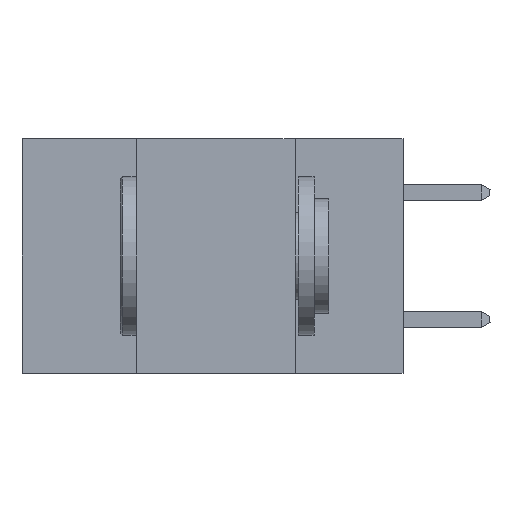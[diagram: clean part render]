
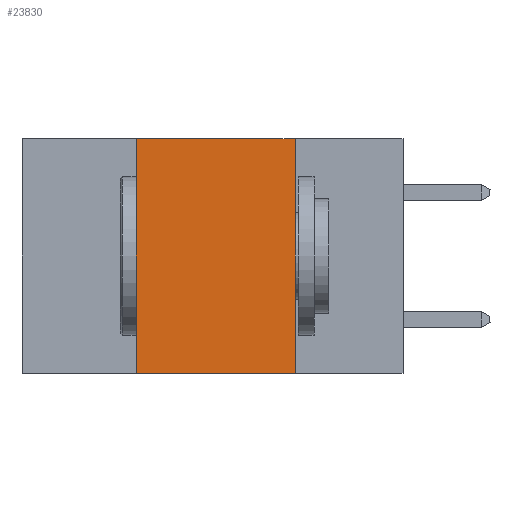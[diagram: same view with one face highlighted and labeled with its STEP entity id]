
A CAD part, left-side view. The second image highlights one B-rep face of the part: STEP entity #23830.
In plain terms, the highlighted planar face has unit normal (-1, 0, 0).
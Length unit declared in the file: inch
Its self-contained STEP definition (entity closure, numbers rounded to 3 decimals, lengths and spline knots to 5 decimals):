
#4 = ORIENTED_EDGE ( 'NONE', *, *, #18553, .F. ) ;
#138 = VECTOR ( 'NONE', #7276, 39.37008 ) ;
#369 = CARTESIAN_POINT ( 'NONE',  ( 0., 0.6, 0. ) ) ;
#420 = CARTESIAN_POINT ( 'NONE',  ( 0., 0.17, -0.37 ) ) ;
#620 = ORIENTED_EDGE ( 'NONE', *, *, #16560, .F. ) ;
#882 = AXIS2_PLACEMENT_3D ( 'NONE', #369, #13523, #2316 ) ;
#1953 = DIRECTION ( 'NONE',  ( 0., 0., -1. ) ) ;
#2316 = DIRECTION ( 'NONE',  ( 0., 0., -1. ) ) ;
#2868 = LINE ( 'NONE', #19048, #3470 ) ;
#3470 = VECTOR ( 'NONE', #17122, 39.37008 ) ;
#3938 = CARTESIAN_POINT ( 'NONE',  ( 0., 0.42, 0. ) ) ;
#5701 = ORIENTED_EDGE ( 'NONE', *, *, #21116, .F. ) ;
#7008 = CARTESIAN_POINT ( 'NONE',  ( 0., 0.42, -0.37 ) ) ;
#7276 = DIRECTION ( 'NONE',  ( 0., 0., 1. ) ) ;
#9091 = VERTEX_POINT ( 'NONE', #7008 ) ;
#9816 = PLANE ( 'NONE',  #882 ) ;
#12121 = VERTEX_POINT ( 'NONE', #19493 ) ;
#13065 = EDGE_LOOP ( 'NONE', ( #4, #620, #5701, #20998 ) ) ;
#13105 = CARTESIAN_POINT ( 'NONE',  ( 0., 0.17, 0. ) ) ;
#13523 = DIRECTION ( 'NONE',  ( 1., 0., 0. ) ) ;
#13578 = FACE_OUTER_BOUND ( 'NONE', #13065, .T. ) ;
#13583 = LINE ( 'NONE', #15158, #22710 ) ;
#13799 = VERTEX_POINT ( 'NONE', #3938 ) ;
#14712 = CARTESIAN_POINT ( 'NONE',  ( 0., 0.42, 0. ) ) ;
#15158 = CARTESIAN_POINT ( 'NONE',  ( 0., 0.6, 0. ) ) ;
#15700 = LINE ( 'NONE', #14712, #138 ) ;
#16560 = EDGE_CURVE ( 'NONE', #13799, #12121, #13583, .T. ) ;
#16988 = DIRECTION ( 'NONE',  ( 0., -1., 0. ) ) ;
#17122 = DIRECTION ( 'NONE',  ( 0., -1., 0. ) ) ;
#18060 = VECTOR ( 'NONE', #1953, 39.37008 ) ;
#18553 = EDGE_CURVE ( 'NONE', #12121, #20566, #23457, .T. ) ;
#19048 = CARTESIAN_POINT ( 'NONE',  ( 0., 0.6, -0.37 ) ) ;
#19493 = CARTESIAN_POINT ( 'NONE',  ( 0., 0.17, 0. ) ) ;
#20566 = VERTEX_POINT ( 'NONE', #420 ) ;
#20998 = ORIENTED_EDGE ( 'NONE', *, *, #21250, .T. ) ;
#21116 = EDGE_CURVE ( 'NONE', #9091, #13799, #15700, .T. ) ;
#21250 = EDGE_CURVE ( 'NONE', #9091, #20566, #2868, .T. ) ;
#22710 = VECTOR ( 'NONE', #16988, 39.37008 ) ;
#23457 = LINE ( 'NONE', #13105, #18060 ) ;
#23830 = ADVANCED_FACE ( 'NONE', ( #13578 ), #9816, .F. ) ;
